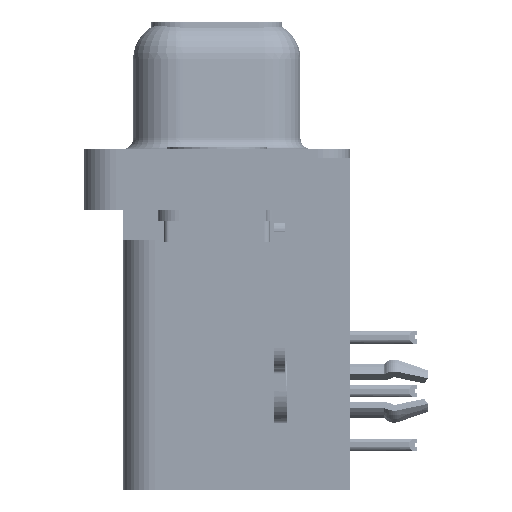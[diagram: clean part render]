
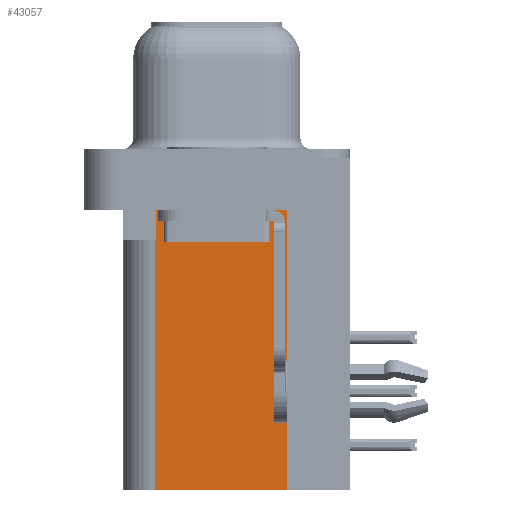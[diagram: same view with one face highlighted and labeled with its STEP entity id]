
A CAD part, left-side view. The second image highlights one B-rep face of the part: STEP entity #43057.
In plain terms, the highlighted planar face has unit normal (-1, 0, 0).
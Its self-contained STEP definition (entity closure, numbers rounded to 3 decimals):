
#3 = EDGE_CURVE ( 'NONE', #32391, #8196, #13689, .T. ) ;
#63 = EDGE_CURVE ( 'NONE', #32391, #36777, #13406, .T. ) ;
#517 = DIRECTION ( 'NONE',  ( 0., 0., -1. ) ) ;
#783 = CARTESIAN_POINT ( 'NONE',  ( 3.7, 2.895, -2.5 ) ) ;
#2448 = CARTESIAN_POINT ( 'NONE',  ( 3.7, -3.295, -15.7 ) ) ;
#2612 = CARTESIAN_POINT ( 'NONE',  ( 3.7, -3.295, -15.7 ) ) ;
#2915 = DIRECTION ( 'NONE',  ( 0., 0., 1. ) ) ;
#4310 = AXIS2_PLACEMENT_3D ( 'NONE', #10577, #14125, #38260 ) ;
#5130 = VERTEX_POINT ( 'NONE', #14185 ) ;
#5390 = CARTESIAN_POINT ( 'NONE',  ( 3.7, -3.295, -15.7 ) ) ;
#5945 = VERTEX_POINT ( 'NONE', #8830 ) ;
#7950 = CARTESIAN_POINT ( 'NONE',  ( 3.7, 0., -3.9 ) ) ;
#8135 = ORIENTED_EDGE ( 'NONE', *, *, #3, .F. ) ;
#8196 = VERTEX_POINT ( 'NONE', #42254 ) ;
#8830 = CARTESIAN_POINT ( 'NONE',  ( 3.7, 2.925, -3.9 ) ) ;
#10577 = CARTESIAN_POINT ( 'NONE',  ( 3.7, -3.295, -15.7 ) ) ;
#11028 = LINE ( 'NONE', #31933, #19317 ) ;
#11341 = LINE ( 'NONE', #41869, #29000 ) ;
#13387 = LINE ( 'NONE', #27802, #30902 ) ;
#13406 = LINE ( 'NONE', #2612, #13448 ) ;
#13448 = VECTOR ( 'NONE', #2915, 1000. ) ;
#13636 = VECTOR ( 'NONE', #14809, 1000. ) ;
#13689 = LINE ( 'NONE', #5390, #13636 ) ;
#14125 = DIRECTION ( 'NONE',  ( 1., 0., 0. ) ) ;
#14185 = CARTESIAN_POINT ( 'NONE',  ( 3.7, 2.895, -3.9 ) ) ;
#14809 = DIRECTION ( 'NONE',  ( 0., 1., 0. ) ) ;
#16045 = EDGE_LOOP ( 'NONE', ( #20405, #17999, #39083, #41561, #8135, #25527 ) ) ;
#17681 = VECTOR ( 'NONE', #42476, 1000. ) ;
#17999 = ORIENTED_EDGE ( 'NONE', *, *, #26438, .T. ) ;
#19317 = VECTOR ( 'NONE', #25279, 1000. ) ;
#19809 = VERTEX_POINT ( 'NONE', #783 ) ;
#20405 = ORIENTED_EDGE ( 'NONE', *, *, #23493, .T. ) ;
#23493 = EDGE_CURVE ( 'NONE', #36777, #19809, #11028, .T. ) ;
#24701 = PLANE ( 'NONE',  #4310 ) ;
#25279 = DIRECTION ( 'NONE',  ( 0., 1., 0. ) ) ;
#25527 = ORIENTED_EDGE ( 'NONE', *, *, #63, .T. ) ;
#26438 = EDGE_CURVE ( 'NONE', #19809, #5130, #11341, .T. ) ;
#27802 = CARTESIAN_POINT ( 'NONE',  ( 3.7, 2.925, -15.7 ) ) ;
#28611 = EDGE_CURVE ( 'NONE', #5130, #5945, #37043, .T. ) ;
#29000 = VECTOR ( 'NONE', #517, 1000. ) ;
#30902 = VECTOR ( 'NONE', #31142, 1000. ) ;
#31142 = DIRECTION ( 'NONE',  ( 0., 0., 1. ) ) ;
#31933 = CARTESIAN_POINT ( 'NONE',  ( 3.7, -3.295, -2.5 ) ) ;
#32391 = VERTEX_POINT ( 'NONE', #2448 ) ;
#36777 = VERTEX_POINT ( 'NONE', #42078 ) ;
#37043 = LINE ( 'NONE', #7950, #17681 ) ;
#37647 = FACE_OUTER_BOUND ( 'NONE', #16045, .T. ) ;
#38260 = DIRECTION ( 'NONE',  ( 0., 0., -1. ) ) ;
#39083 = ORIENTED_EDGE ( 'NONE', *, *, #28611, .T. ) ;
#41561 = ORIENTED_EDGE ( 'NONE', *, *, #42345, .F. ) ;
#41869 = CARTESIAN_POINT ( 'NONE',  ( 3.7, 2.895, -3.9 ) ) ;
#42078 = CARTESIAN_POINT ( 'NONE',  ( 3.7, -3.295, -2.5 ) ) ;
#42254 = CARTESIAN_POINT ( 'NONE',  ( 3.7, 2.925, -15.7 ) ) ;
#42345 = EDGE_CURVE ( 'NONE', #8196, #5945, #13387, .T. ) ;
#42476 = DIRECTION ( 'NONE',  ( 0., 1., 0. ) ) ;
#43057 = ADVANCED_FACE ( 'NONE', ( #37647 ), #24701, .F. ) ;
